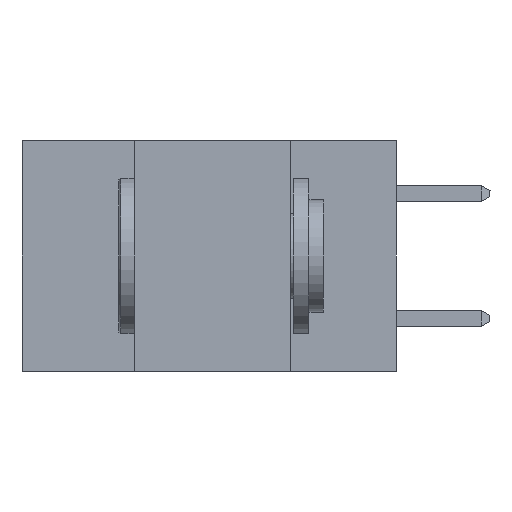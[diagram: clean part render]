
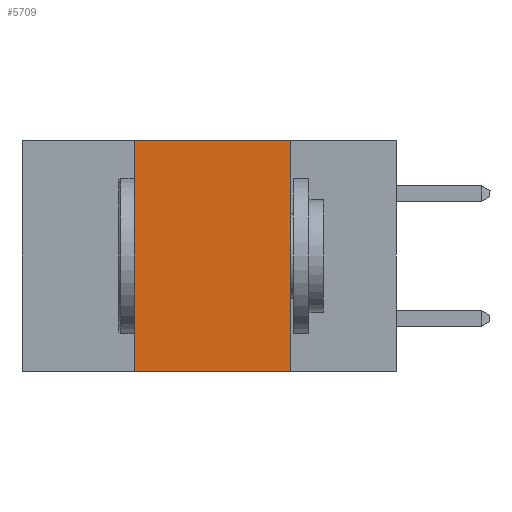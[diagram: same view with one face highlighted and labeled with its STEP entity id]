
A CAD part, left-side view. The second image highlights one B-rep face of the part: STEP entity #5709.
In plain terms, the highlighted planar face has unit normal (-1, 0, 0).
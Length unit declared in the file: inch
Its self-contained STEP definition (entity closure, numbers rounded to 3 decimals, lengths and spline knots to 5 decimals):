
#55 = CARTESIAN_POINT ( 'NONE',  ( 0., 0.17, 0. ) ) ;
#391 = DIRECTION ( 'NONE',  ( 0., 0., -1. ) ) ;
#933 = DIRECTION ( 'NONE',  ( 0., -1., 0. ) ) ;
#1065 = VERTEX_POINT ( 'NONE', #9934 ) ;
#1996 = CARTESIAN_POINT ( 'NONE',  ( 0., 0.6, 0. ) ) ;
#2010 = ORIENTED_EDGE ( 'NONE', *, *, #7392, .T. ) ;
#2271 = DIRECTION ( 'NONE',  ( 0., 0., -1. ) ) ;
#2426 = DIRECTION ( 'NONE',  ( 1., 0., 0. ) ) ;
#2849 = CARTESIAN_POINT ( 'NONE',  ( 0., 0.42, -0.37 ) ) ;
#2901 = VECTOR ( 'NONE', #933, 39.37008 ) ;
#3064 = VERTEX_POINT ( 'NONE', #10019 ) ;
#3761 = LINE ( 'NONE', #10636, #8836 ) ;
#3793 = PLANE ( 'NONE',  #6353 ) ;
#5459 = EDGE_CURVE ( 'NONE', #12202, #3064, #7029, .T. ) ;
#5589 = DIRECTION ( 'NONE',  ( 0., 0., 1. ) ) ;
#5709 = ADVANCED_FACE ( 'NONE', ( #6561 ), #3793, .F. ) ;
#6031 = CARTESIAN_POINT ( 'NONE',  ( 0., 0.17, 0. ) ) ;
#6353 = AXIS2_PLACEMENT_3D ( 'NONE', #1996, #2426, #2271 ) ;
#6561 = FACE_OUTER_BOUND ( 'NONE', #10866, .T. ) ;
#6737 = VECTOR ( 'NONE', #12563, 39.37008 ) ;
#7029 = LINE ( 'NONE', #55, #9397 ) ;
#7187 = CARTESIAN_POINT ( 'NONE',  ( 0., 0.6, -0.37 ) ) ;
#7392 = EDGE_CURVE ( 'NONE', #11506, #3064, #11099, .T. ) ;
#8190 = EDGE_CURVE ( 'NONE', #11506, #1065, #3761, .T. ) ;
#8836 = VECTOR ( 'NONE', #5589, 39.37008 ) ;
#9397 = VECTOR ( 'NONE', #391, 39.37008 ) ;
#9934 = CARTESIAN_POINT ( 'NONE',  ( 0., 0.42, 0. ) ) ;
#10010 = EDGE_CURVE ( 'NONE', #1065, #12202, #11851, .T. ) ;
#10019 = CARTESIAN_POINT ( 'NONE',  ( 0., 0.17, -0.37 ) ) ;
#10500 = ORIENTED_EDGE ( 'NONE', *, *, #10010, .F. ) ;
#10636 = CARTESIAN_POINT ( 'NONE',  ( 0., 0.42, 0. ) ) ;
#10866 = EDGE_LOOP ( 'NONE', ( #11847, #10500, #10978, #2010 ) ) ;
#10978 = ORIENTED_EDGE ( 'NONE', *, *, #8190, .F. ) ;
#11099 = LINE ( 'NONE', #7187, #2901 ) ;
#11506 = VERTEX_POINT ( 'NONE', #2849 ) ;
#11563 = CARTESIAN_POINT ( 'NONE',  ( 0., 0.6, 0. ) ) ;
#11847 = ORIENTED_EDGE ( 'NONE', *, *, #5459, .F. ) ;
#11851 = LINE ( 'NONE', #11563, #6737 ) ;
#12202 = VERTEX_POINT ( 'NONE', #6031 ) ;
#12563 = DIRECTION ( 'NONE',  ( 0., -1., 0. ) ) ;
